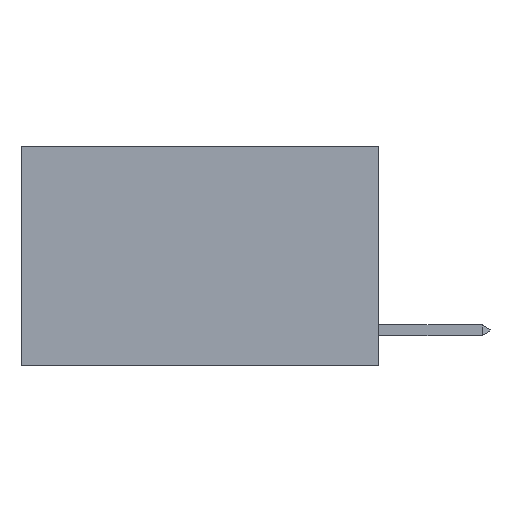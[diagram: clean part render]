
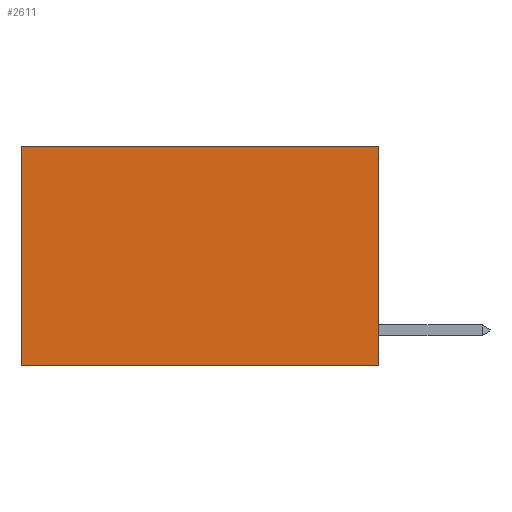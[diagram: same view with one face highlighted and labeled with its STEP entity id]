
A CAD part, left-side view. The second image highlights one B-rep face of the part: STEP entity #2611.
In plain terms, the highlighted planar face has unit normal (-1, 0, 0).
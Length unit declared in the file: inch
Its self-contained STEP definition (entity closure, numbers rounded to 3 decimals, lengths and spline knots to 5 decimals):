
#225 = ORIENTED_EDGE ( 'NONE', *, *, #5262, .T. ) ;
#450 = ORIENTED_EDGE ( 'NONE', *, *, #1113, .F. ) ;
#648 = CARTESIAN_POINT ( 'NONE',  ( 0.2625, 0.6, 0. ) ) ;
#1062 = EDGE_LOOP ( 'NONE', ( #6617, #8300, #450, #225 ) ) ;
#1113 = EDGE_CURVE ( 'NONE', #1639, #2408, #2614, .T. ) ;
#1246 = PLANE ( 'NONE',  #4398 ) ;
#1247 = VERTEX_POINT ( 'NONE', #5452 ) ;
#1292 = EDGE_CURVE ( 'NONE', #2408, #4332, #7600, .T. ) ;
#1430 = CARTESIAN_POINT ( 'NONE',  ( 0.2625, 0., 0. ) ) ;
#1639 = VERTEX_POINT ( 'NONE', #1430 ) ;
#1700 = DIRECTION ( 'NONE',  ( 0., 0., -1. ) ) ;
#2255 = CARTESIAN_POINT ( 'NONE',  ( 0.2625, 0., 0. ) ) ;
#2408 = VERTEX_POINT ( 'NONE', #7996 ) ;
#2611 = ADVANCED_FACE ( 'NONE', ( #7871 ), #1246, .F. ) ;
#2614 = LINE ( 'NONE', #6276, #4231 ) ;
#2785 = DIRECTION ( 'NONE',  ( 0., 0., -1. ) ) ;
#3136 = VECTOR ( 'NONE', #7845, 39.37008 ) ;
#3416 = EDGE_CURVE ( 'NONE', #1247, #4332, #4907, .T. ) ;
#4231 = VECTOR ( 'NONE', #1700, 39.37008 ) ;
#4332 = VERTEX_POINT ( 'NONE', #6402 ) ;
#4398 = AXIS2_PLACEMENT_3D ( 'NONE', #7626, #6540, #2785 ) ;
#4907 = LINE ( 'NONE', #648, #7967 ) ;
#5060 = LINE ( 'NONE', #2255, #3136 ) ;
#5262 = EDGE_CURVE ( 'NONE', #1639, #1247, #5060, .T. ) ;
#5343 = DIRECTION ( 'NONE',  ( 0., 1., 0. ) ) ;
#5452 = CARTESIAN_POINT ( 'NONE',  ( 0.2625, 0.6, 0. ) ) ;
#5511 = DIRECTION ( 'NONE',  ( 0., 0., -1. ) ) ;
#5745 = CARTESIAN_POINT ( 'NONE',  ( 0.2625, 0., -0.37 ) ) ;
#6276 = CARTESIAN_POINT ( 'NONE',  ( 0.2625, 0., 0. ) ) ;
#6402 = CARTESIAN_POINT ( 'NONE',  ( 0.2625, 0.6, -0.37 ) ) ;
#6540 = DIRECTION ( 'NONE',  ( 1., 0., 0. ) ) ;
#6617 = ORIENTED_EDGE ( 'NONE', *, *, #3416, .T. ) ;
#7426 = VECTOR ( 'NONE', #5343, 39.37008 ) ;
#7600 = LINE ( 'NONE', #5745, #7426 ) ;
#7626 = CARTESIAN_POINT ( 'NONE',  ( 0.2625, 0., 0. ) ) ;
#7845 = DIRECTION ( 'NONE',  ( 0., 1., 0. ) ) ;
#7871 = FACE_OUTER_BOUND ( 'NONE', #1062, .T. ) ;
#7967 = VECTOR ( 'NONE', #5511, 39.37008 ) ;
#7996 = CARTESIAN_POINT ( 'NONE',  ( 0.2625, 0., -0.37 ) ) ;
#8300 = ORIENTED_EDGE ( 'NONE', *, *, #1292, .F. ) ;
